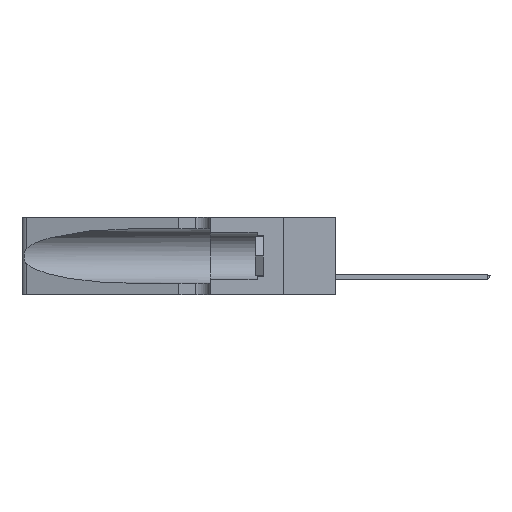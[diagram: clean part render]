
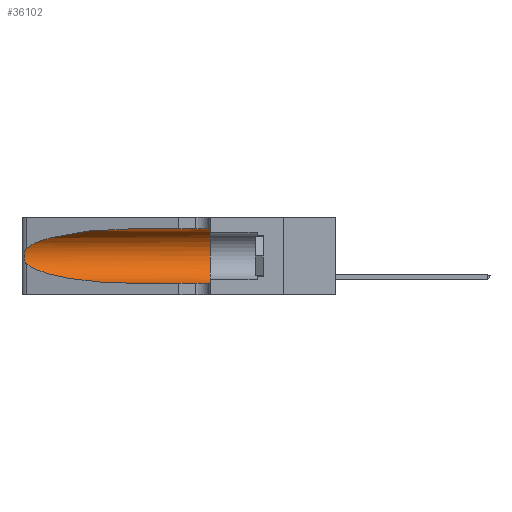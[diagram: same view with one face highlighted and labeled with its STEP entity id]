
A CAD part, left-side view. The second image highlights one B-rep face of the part: STEP entity #36102.
In plain terms, the highlighted cylindrical face has radius 3.308 mm (diameter 6.617 mm), a partial arc.
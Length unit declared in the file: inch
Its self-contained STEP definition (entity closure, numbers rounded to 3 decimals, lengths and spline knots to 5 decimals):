
#1508 = CARTESIAN_POINT ( 'NONE',  ( 0.25487, 1.22718, 0.22369 ) ) ;
#2569 = CARTESIAN_POINT ( 'NONE',  ( 0.1305, 1.61858, 0.185 ) ) ;
#3159 = ORIENTED_EDGE ( 'NONE', *, *, #12950, .T. ) ;
#3890 = EDGE_CURVE ( 'NONE', #24838, #13056, #22806, .T. ) ;
#4185 = EDGE_CURVE ( 'NONE', #24523, #17330, #25209, .T. ) ;
#4654 = CIRCLE ( 'NONE', #38434, 0.13025 ) ;
#5591 = FACE_OUTER_BOUND ( 'NONE', #8910, .T. ) ;
#6824 = B_SPLINE_CURVE_WITH_KNOTS ( 'NONE', 3,
 ( #22057, #15852, #7320, #30917, #10403, #28075, #31184, #22191, #10275, #31054, #13276, #16253, #19496, #25501 ),
 .UNSPECIFIED., .F., .F.,
 ( 4, 2, 2, 2, 2, 2, 4 ),
 ( 0., 0.00027, 0.00053, 0.00107, 0.0016, 0.00187, 0.00214 ),
 .UNSPECIFIED. ) ;
#7320 = CARTESIAN_POINT ( 'NONE',  ( 0.25639, 1.23184, 0.21858 ) ) ;
#8910 = EDGE_LOOP ( 'NONE', ( #13564, #3159, #32016, #38432, #18889, #36322 ) ) ;
#9812 = DIRECTION ( 'NONE',  ( 0., 0., 1. ) ) ;
#9944 = CARTESIAN_POINT ( 'NONE',  ( 0.1305, 0.72297, 0.31525 ) ) ;
#10275 = CARTESIAN_POINT ( 'NONE',  ( 0.26017, 1.23833, 0.17102 ) ) ;
#10403 = CARTESIAN_POINT ( 'NONE',  ( 0.25854, 1.2359, 0.20912 ) ) ;
#10899 = CARTESIAN_POINT ( 'NONE',  ( 0.1305, 0.35, 0.05475 ) ) ;
#11302 = EDGE_CURVE ( 'NONE', #13257, #17330, #4654, .T. ) ;
#12828 = LINE ( 'NONE', #38411, #37014 ) ;
#12838 = AXIS2_PLACEMENT_3D ( 'NONE', #2569, #29695, #23590 ) ;
#12950 = EDGE_CURVE ( 'NONE', #13056, #22974, #6824, .T. ) ;
#12963 = CARTESIAN_POINT ( 'NONE',  ( 0.2373, 1.15595, 0.28018 ) ) ;
#13056 = VERTEX_POINT ( 'NONE', #21270 ) ;
#13257 = VERTEX_POINT ( 'NONE', #37062 ) ;
#13276 = CARTESIAN_POINT ( 'NONE',  ( 0.25789, 1.23486, 0.15765 ) ) ;
#13564 = ORIENTED_EDGE ( 'NONE', *, *, #3890, .T. ) ;
#15852 = CARTESIAN_POINT ( 'NONE',  ( 0.25555, 1.22994, 0.2215 ) ) ;
#16253 = CARTESIAN_POINT ( 'NONE',  ( 0.25639, 1.23186, 0.15144 ) ) ;
#17330 = VERTEX_POINT ( 'NONE', #10899 ) ;
#17567 = CARTESIAN_POINT ( 'NONE',  ( 0.1305, 0.72297, 0.05475 ) ) ;
#18889 = ORIENTED_EDGE ( 'NONE', *, *, #11302, .F. ) ;
#19143 = VECTOR ( 'NONE', #34634, 39.37008 ) ;
#19285 = CARTESIAN_POINT ( 'NONE',  ( 0.1305, 0.35, 0.185 ) ) ;
#19457 = CYLINDRICAL_SURFACE ( 'NONE', #12838, 0.13025 ) ;
#19496 = CARTESIAN_POINT ( 'NONE',  ( 0.25555, 1.22993, 0.14849 ) ) ;
#21270 = CARTESIAN_POINT ( 'NONE',  ( 0.25487, 1.22718, 0.22369 ) ) ;
#21588 = CARTESIAN_POINT ( 'NONE',  ( 0.18966, 0.96281, 0.05475 ) ) ;
#22057 = CARTESIAN_POINT ( 'NONE',  ( 0.25487, 1.22718, 0.22369 ) ) ;
#22191 = CARTESIAN_POINT ( 'NONE',  ( 0.26075, 1.23896, 0.178 ) ) ;
#22468 = CARTESIAN_POINT ( 'NONE',  ( 0.1305, 0.72297, 0.31525 ) ) ;
#22806 =( BOUNDED_CURVE ( )  B_SPLINE_CURVE ( 3, ( #9944, #25293, #12963, #1508 ),
 .UNSPECIFIED., .F., .T. ) 
 B_SPLINE_CURVE_WITH_KNOTS ( ( 4, 4 ),
 ( 1.5708, 2.84003 ),
 .UNSPECIFIED. ) 
 CURVE ( )  GEOMETRIC_REPRESENTATION_ITEM ( )  RATIONAL_B_SPLINE_CURVE ( ( 1., 0.87, 0.87, 1. ) ) 
 REPRESENTATION_ITEM ( '' )  );
#22974 = VERTEX_POINT ( 'NONE', #25712 ) ;
#23590 = DIRECTION ( 'NONE',  ( 0., 0., -1. ) ) ;
#23935 = DIRECTION ( 'NONE',  ( 0., -1., 0. ) ) ;
#24523 = VERTEX_POINT ( 'NONE', #17567 ) ;
#24838 = VERTEX_POINT ( 'NONE', #22468 ) ;
#25138 = CARTESIAN_POINT ( 'NONE',  ( 0.2373, 1.15595, 0.08982 ) ) ;
#25209 = LINE ( 'NONE', #37644, #19143 ) ;
#25293 = CARTESIAN_POINT ( 'NONE',  ( 0.18966, 0.96281, 0.31525 ) ) ;
#25501 = CARTESIAN_POINT ( 'NONE',  ( 0.25487, 1.22718, 0.14631 ) ) ;
#25712 = CARTESIAN_POINT ( 'NONE',  ( 0.25487, 1.22718, 0.14631 ) ) ;
#28075 = CARTESIAN_POINT ( 'NONE',  ( 0.26018, 1.23835, 0.19895 ) ) ;
#29695 = DIRECTION ( 'NONE',  ( 0., -1., 0. ) ) ;
#30485 = EDGE_CURVE ( 'NONE', #24838, #13257, #12828, .T. ) ;
#30846 = CARTESIAN_POINT ( 'NONE',  ( 0.25487, 1.22718, 0.14631 ) ) ;
#30917 = CARTESIAN_POINT ( 'NONE',  ( 0.25787, 1.23484, 0.2124 ) ) ;
#31054 = CARTESIAN_POINT ( 'NONE',  ( 0.25856, 1.23593, 0.16098 ) ) ;
#31184 = CARTESIAN_POINT ( 'NONE',  ( 0.26075, 1.23896, 0.19203 ) ) ;
#32016 = ORIENTED_EDGE ( 'NONE', *, *, #32935, .T. ) ;
#32935 = EDGE_CURVE ( 'NONE', #22974, #24523, #34988, .T. ) ;
#33585 = DIRECTION ( 'NONE',  ( 0., 1., 0. ) ) ;
#34634 = DIRECTION ( 'NONE',  ( 0., -1., 0. ) ) ;
#34988 =( BOUNDED_CURVE ( )  B_SPLINE_CURVE ( 3, ( #30846, #25138, #21588, #36865 ),
 .UNSPECIFIED., .F., .F. ) 
 B_SPLINE_CURVE_WITH_KNOTS ( ( 4, 4 ),
 ( 3.44316, 4.71239 ),
 .UNSPECIFIED. ) 
 CURVE ( )  GEOMETRIC_REPRESENTATION_ITEM ( )  RATIONAL_B_SPLINE_CURVE ( ( 1., 0.87, 0.87, 1. ) ) 
 REPRESENTATION_ITEM ( '' )  );
#36102 = ADVANCED_FACE ( 'NONE', ( #5591 ), #19457, .F. ) ;
#36322 = ORIENTED_EDGE ( 'NONE', *, *, #30485, .F. ) ;
#36865 = CARTESIAN_POINT ( 'NONE',  ( 0.1305, 0.72297, 0.05475 ) ) ;
#37014 = VECTOR ( 'NONE', #23935, 39.37008 ) ;
#37062 = CARTESIAN_POINT ( 'NONE',  ( 0.1305, 0.35, 0.31525 ) ) ;
#37644 = CARTESIAN_POINT ( 'NONE',  ( 0.1305, 1.61858, 0.05475 ) ) ;
#38411 = CARTESIAN_POINT ( 'NONE',  ( 0.1305, 1.61858, 0.31525 ) ) ;
#38432 = ORIENTED_EDGE ( 'NONE', *, *, #4185, .T. ) ;
#38434 = AXIS2_PLACEMENT_3D ( 'NONE', #19285, #33585, #9812 ) ;
